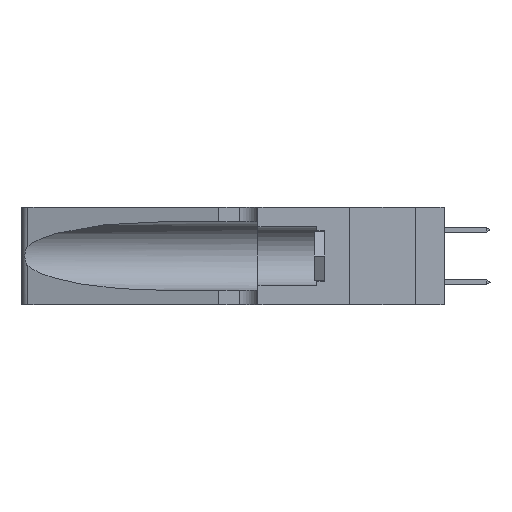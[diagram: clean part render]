
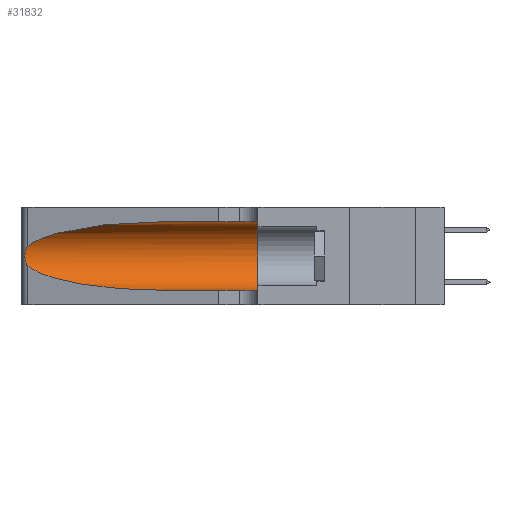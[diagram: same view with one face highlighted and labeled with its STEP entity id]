
A CAD part, left-side view. The second image highlights one B-rep face of the part: STEP entity #31832.
In plain terms, the highlighted cylindrical face has radius 3.308 mm (diameter 6.617 mm), a partial arc.
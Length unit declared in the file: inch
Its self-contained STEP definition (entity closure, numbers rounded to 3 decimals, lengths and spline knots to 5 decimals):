
#101 = CARTESIAN_POINT ( 'NONE',  ( 0.25856, 1.23593, 0.16098 ) ) ;
#165 = AXIS2_PLACEMENT_3D ( 'NONE', #7032, #32737, #12743 ) ;
#870 = DIRECTION ( 'NONE',  ( 0., 0., 1. ) ) ;
#1398 = CARTESIAN_POINT ( 'NONE',  ( 0.2373, 1.15595, 0.28018 ) ) ;
#1858 = B_SPLINE_CURVE_WITH_KNOTS ( 'NONE', 3,
 ( #7756, #20397, #2596, #25452, #10305, #27937, #12854, #30456, #15401, #101, #17951, #2707, #20512, #5282 ),
 .UNSPECIFIED., .F., .F.,
 ( 4, 2, 2, 2, 2, 2, 4 ),
 ( 0., 0.00027, 0.00053, 0.00107, 0.0016, 0.00187, 0.00214 ),
 .UNSPECIFIED. ) ;
#2080 = VERTEX_POINT ( 'NONE', #9728 ) ;
#2596 = CARTESIAN_POINT ( 'NONE',  ( 0.25639, 1.23184, 0.21858 ) ) ;
#2707 = CARTESIAN_POINT ( 'NONE',  ( 0.25639, 1.23186, 0.15144 ) ) ;
#4318 = CIRCLE ( 'NONE', #26645, 0.13025 ) ;
#5182 = EDGE_CURVE ( 'NONE', #7871, #2080, #28819, .T. ) ;
#5282 = CARTESIAN_POINT ( 'NONE',  ( 0.25487, 1.22718, 0.14631 ) ) ;
#6028 = ORIENTED_EDGE ( 'NONE', *, *, #8744, .T. ) ;
#6476 = CARTESIAN_POINT ( 'NONE',  ( 0.18966, 0.96281, 0.31525 ) ) ;
#6591 = ORIENTED_EDGE ( 'NONE', *, *, #5182, .T. ) ;
#7032 = CARTESIAN_POINT ( 'NONE',  ( 0.1305, 1.61858, 0.185 ) ) ;
#7115 = EDGE_LOOP ( 'NONE', ( #29614, #6028, #23791, #6591, #8602, #14837 ) ) ;
#7237 = CARTESIAN_POINT ( 'NONE',  ( 0.25487, 1.22718, 0.14631 ) ) ;
#7738 = CYLINDRICAL_SURFACE ( 'NONE', #165, 0.13025 ) ;
#7756 = CARTESIAN_POINT ( 'NONE',  ( 0.25487, 1.22718, 0.22369 ) ) ;
#7871 = VERTEX_POINT ( 'NONE', #9227 ) ;
#8529 = FACE_OUTER_BOUND ( 'NONE', #7115, .T. ) ;
#8602 = ORIENTED_EDGE ( 'NONE', *, *, #24637, .F. ) ;
#8744 = EDGE_CURVE ( 'NONE', #12493, #30540, #1858, .T. ) ;
#9227 = CARTESIAN_POINT ( 'NONE',  ( 0.1305, 0.72297, 0.05475 ) ) ;
#9290 =( BOUNDED_CURVE ( )  B_SPLINE_CURVE ( 3, ( #11586, #6476, #1398, #19236 ),
 .UNSPECIFIED., .F., .F. ) 
 B_SPLINE_CURVE_WITH_KNOTS ( ( 4, 4 ),
 ( 1.5708, 2.84003 ),
 .UNSPECIFIED. ) 
 CURVE ( )  GEOMETRIC_REPRESENTATION_ITEM ( )  RATIONAL_B_SPLINE_CURVE ( ( 1., 0.87, 0.87, 1. ) ) 
 REPRESENTATION_ITEM ( '' )  );
#9728 = CARTESIAN_POINT ( 'NONE',  ( 0.1305, 0.35, 0.05475 ) ) ;
#10305 = CARTESIAN_POINT ( 'NONE',  ( 0.25854, 1.2359, 0.20912 ) ) ;
#11337 = VECTOR ( 'NONE', #19391, 39.37008 ) ;
#11586 = CARTESIAN_POINT ( 'NONE',  ( 0.1305, 0.72297, 0.31525 ) ) ;
#12124 = LINE ( 'NONE', #14416, #11337 ) ;
#12493 = VERTEX_POINT ( 'NONE', #22444 ) ;
#12743 = DIRECTION ( 'NONE',  ( 0., 0., -1. ) ) ;
#12854 = CARTESIAN_POINT ( 'NONE',  ( 0.26075, 1.23896, 0.19203 ) ) ;
#12931 = VERTEX_POINT ( 'NONE', #19424 ) ;
#14416 = CARTESIAN_POINT ( 'NONE',  ( 0.1305, 1.61858, 0.31525 ) ) ;
#14837 = ORIENTED_EDGE ( 'NONE', *, *, #18870, .F. ) ;
#14896 = CARTESIAN_POINT ( 'NONE',  ( 0.18966, 0.96281, 0.05475 ) ) ;
#15401 = CARTESIAN_POINT ( 'NONE',  ( 0.26017, 1.23833, 0.17102 ) ) ;
#15428 = VECTOR ( 'NONE', #18125, 39.37008 ) ;
#16159 = DIRECTION ( 'NONE',  ( 0., 1., 0. ) ) ;
#17951 = CARTESIAN_POINT ( 'NONE',  ( 0.25789, 1.23486, 0.15765 ) ) ;
#18125 = DIRECTION ( 'NONE',  ( 0., -1., 0. ) ) ;
#18870 = EDGE_CURVE ( 'NONE', #25141, #12931, #12124, .T. ) ;
#19236 = CARTESIAN_POINT ( 'NONE',  ( 0.25487, 1.22718, 0.22369 ) ) ;
#19391 = DIRECTION ( 'NONE',  ( 0., -1., 0. ) ) ;
#19424 = CARTESIAN_POINT ( 'NONE',  ( 0.1305, 0.35, 0.31525 ) ) ;
#20397 = CARTESIAN_POINT ( 'NONE',  ( 0.25555, 1.22994, 0.2215 ) ) ;
#20512 = CARTESIAN_POINT ( 'NONE',  ( 0.25555, 1.22993, 0.14849 ) ) ;
#22444 = CARTESIAN_POINT ( 'NONE',  ( 0.25487, 1.22718, 0.22369 ) ) ;
#23791 = ORIENTED_EDGE ( 'NONE', *, *, #28026, .T. ) ;
#24218 = EDGE_CURVE ( 'NONE', #25141, #12493, #9290, .T. ) ;
#24510 =( BOUNDED_CURVE ( )  B_SPLINE_CURVE ( 3, ( #7237, #27436, #14896, #32448 ),
 .UNSPECIFIED., .F., .F. ) 
 B_SPLINE_CURVE_WITH_KNOTS ( ( 4, 4 ),
 ( 3.44316, 4.71239 ),
 .UNSPECIFIED. ) 
 CURVE ( )  GEOMETRIC_REPRESENTATION_ITEM ( )  RATIONAL_B_SPLINE_CURVE ( ( 1., 0.87, 0.87, 1. ) ) 
 REPRESENTATION_ITEM ( '' )  );
#24637 = EDGE_CURVE ( 'NONE', #12931, #2080, #4318, .T. ) ;
#25141 = VERTEX_POINT ( 'NONE', #28671 ) ;
#25452 = CARTESIAN_POINT ( 'NONE',  ( 0.25787, 1.23484, 0.2124 ) ) ;
#26645 = AXIS2_PLACEMENT_3D ( 'NONE', #31208, #16159, #870 ) ;
#27436 = CARTESIAN_POINT ( 'NONE',  ( 0.2373, 1.15595, 0.08982 ) ) ;
#27937 = CARTESIAN_POINT ( 'NONE',  ( 0.26018, 1.23835, 0.19895 ) ) ;
#28026 = EDGE_CURVE ( 'NONE', #30540, #7871, #24510, .T. ) ;
#28110 = CARTESIAN_POINT ( 'NONE',  ( 0.1305, 1.61858, 0.05475 ) ) ;
#28671 = CARTESIAN_POINT ( 'NONE',  ( 0.1305, 0.72297, 0.31525 ) ) ;
#28819 = LINE ( 'NONE', #28110, #15428 ) ;
#29614 = ORIENTED_EDGE ( 'NONE', *, *, #24218, .T. ) ;
#30085 = CARTESIAN_POINT ( 'NONE',  ( 0.25487, 1.22718, 0.14631 ) ) ;
#30456 = CARTESIAN_POINT ( 'NONE',  ( 0.26075, 1.23896, 0.178 ) ) ;
#30540 = VERTEX_POINT ( 'NONE', #30085 ) ;
#31208 = CARTESIAN_POINT ( 'NONE',  ( 0.1305, 0.35, 0.185 ) ) ;
#31832 = ADVANCED_FACE ( 'NONE', ( #8529 ), #7738, .F. ) ;
#32448 = CARTESIAN_POINT ( 'NONE',  ( 0.1305, 0.72297, 0.05475 ) ) ;
#32737 = DIRECTION ( 'NONE',  ( 0., -1., 0. ) ) ;
